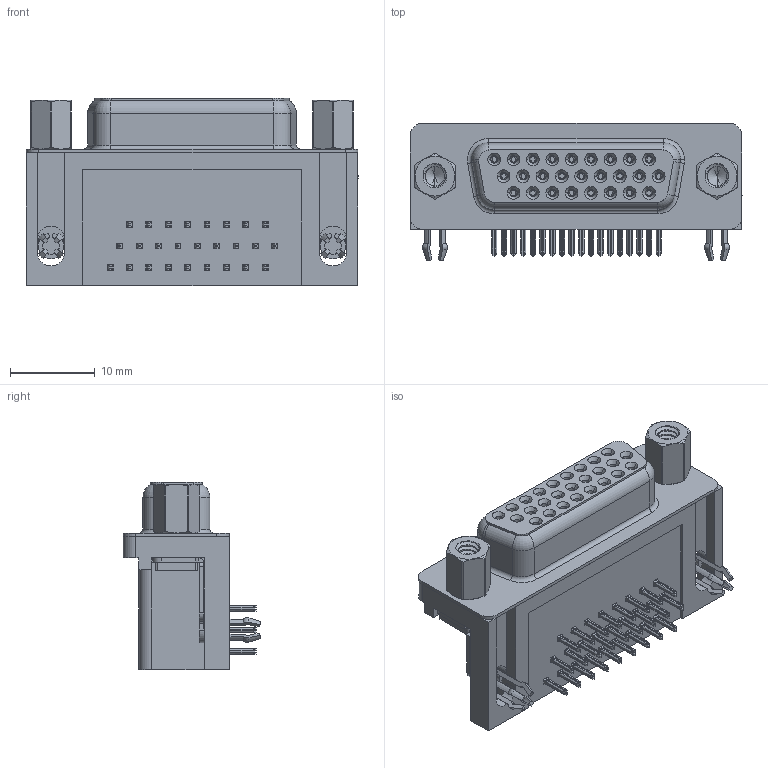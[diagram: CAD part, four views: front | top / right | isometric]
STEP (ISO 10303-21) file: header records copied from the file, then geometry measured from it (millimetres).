
FILE_DESCRIPTION (( 'STEP AP203' ), '1' );
FILE_NAME ('634-026-663-553.STEP', '2018-08-18T04:28:51', ( '' ), ( '' ), 'SwSTEP 2.0', 'SolidWorks 2016', '' );
FILE_SCHEMA (( 'CONFIG_CONTROL_DESIGN' ));
Length unit declared in the file: millimetre
Products named in the file (9): Contact Middle; Contact Top; 4 Prong Board Lock; 4-40 Threaded Rivet; 4-40 Hex Standoff; 634-026-663-553; 634 Housing_26 Socket; 634 Shell_26 Socket; Contact Bottom
Assembly tree (34 placements, depth 2):
  634-026-663-553
    634 Housing_26 Socket
    634 Shell_26 Socket
    Contact Bottom  x8
    Contact Middle  x9
    Contact Top  x9
    4 Prong Board Lock  x2
    4-40 Threaded Rivet  x2
    4-40 Hex Standoff  x2
Bounding box: 39.22 x 16.25 x 22.1 mm (x, y, z)
Volume: 6577.7 mm3; surface area: 9607 mm2
Topology: 34 solids, 34 shells, 4221 faces, 11150 edges, 7022 vertices
Faces by surface type: plane 1835, cylinder 1008, bspline 922, cone 386, torus 70
Entity records: 43035 total; most frequent: CARTESIAN_POINT 15420, ORIENTED_EDGE 5642, DIRECTION 4994, EDGE_CURVE 2821, VERTEX_POINT 1804, VECTOR 1716, LINE 1716, AXIS2_PLACEMENT_3D 1639
